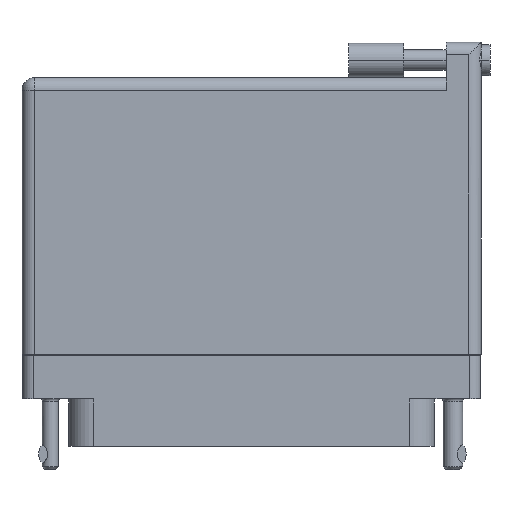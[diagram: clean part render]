
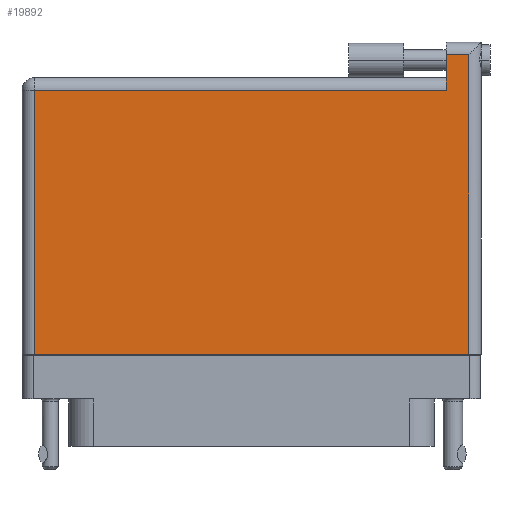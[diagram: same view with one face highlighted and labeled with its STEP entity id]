
A CAD part, front view. The second image highlights one B-rep face of the part: STEP entity #19892.
In plain terms, the highlighted face is planar.
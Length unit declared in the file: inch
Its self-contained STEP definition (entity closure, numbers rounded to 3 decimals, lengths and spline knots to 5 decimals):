
#1408 = CARTESIAN_POINT ( 'NONE',  ( 1.23, 1.666, 0.4495 ) ) ;
#2684 = EDGE_CURVE ( 'NONE', #15771, #12759, #55720, .T. ) ;
#5996 = FACE_OUTER_BOUND ( 'NONE', #47998, .T. ) ;
#6559 = CARTESIAN_POINT ( 'NONE',  ( -1.3, 1.466, 0.4495 ) ) ;
#7021 = EDGE_CURVE ( 'NONE', #54679, #48493, #30972, .T. ) ;
#7186 = VECTOR ( 'NONE', #22180, 39.37008 ) ;
#11133 = VECTOR ( 'NONE', #48648, 39.37008 ) ;
#11405 = CARTESIAN_POINT ( 'NONE',  ( 1.23, 1.596, 0.4495 ) ) ;
#11908 = ORIENTED_EDGE ( 'NONE', *, *, #27529, .T. ) ;
#12759 = VERTEX_POINT ( 'NONE', #29546 ) ;
#13455 = EDGE_CURVE ( 'NONE', #48493, #41974, #55387, .T. ) ;
#15771 = VERTEX_POINT ( 'NONE', #11405 ) ;
#19892 = ADVANCED_FACE ( 'NONE', ( #5996 ), #20481, .F. ) ;
#20481 = PLANE ( 'NONE',  #52859 ) ;
#20877 = ORIENTED_EDGE ( 'NONE', *, *, #7021, .T. ) ;
#22180 = DIRECTION ( 'NONE',  ( -1., 0., 0. ) ) ;
#22475 = ORIENTED_EDGE ( 'NONE', *, *, #58324, .T. ) ;
#27529 = EDGE_CURVE ( 'NONE', #51222, #54679, #41336, .T. ) ;
#28991 = CARTESIAN_POINT ( 'NONE',  ( -1.3, 1.396, 0.4495 ) ) ;
#29499 = CARTESIAN_POINT ( 'NONE',  ( -1.3, -0.1, 0.4495 ) ) ;
#29546 = CARTESIAN_POINT ( 'NONE',  ( 1.103, 1.596, 0.4495 ) ) ;
#29896 = DIRECTION ( 'NONE',  ( 1., 0., 0. ) ) ;
#30972 = LINE ( 'NONE', #33881, #50880 ) ;
#31737 = VECTOR ( 'NONE', #47667, 39.37008 ) ;
#33881 = CARTESIAN_POINT ( 'NONE',  ( -1.23, -0.1, 0.4495 ) ) ;
#38364 = LINE ( 'NONE', #60216, #44228 ) ;
#40346 = CARTESIAN_POINT ( 'NONE',  ( 1.103, 1.396, 0.4495 ) ) ;
#41021 = CARTESIAN_POINT ( 'NONE',  ( -1.23, 1.396, 0.4495 ) ) ;
#41336 = LINE ( 'NONE', #28991, #31737 ) ;
#41974 = VERTEX_POINT ( 'NONE', #44937 ) ;
#42903 = VECTOR ( 'NONE', #29896, 39.37008 ) ;
#43570 = DIRECTION ( 'NONE',  ( 0., -1., 0. ) ) ;
#44228 = VECTOR ( 'NONE', #46209, 39.37008 ) ;
#44307 = ORIENTED_EDGE ( 'NONE', *, *, #13455, .T. ) ;
#44333 = DIRECTION ( 'NONE',  ( -1., 0., 0. ) ) ;
#44937 = CARTESIAN_POINT ( 'NONE',  ( 1.23, -0.1, 0.4495 ) ) ;
#46209 = DIRECTION ( 'NONE',  ( 0., -1., 0. ) ) ;
#47667 = DIRECTION ( 'NONE',  ( -1., 0., 0. ) ) ;
#47998 = EDGE_LOOP ( 'NONE', ( #44307, #58967, #52487, #22475, #11908, #20877 ) ) ;
#48493 = VERTEX_POINT ( 'NONE', #55356 ) ;
#48648 = DIRECTION ( 'NONE',  ( 0., 1., 0. ) ) ;
#50334 = CARTESIAN_POINT ( 'NONE',  ( -1.3, 1.596, 0.4495 ) ) ;
#50776 = LINE ( 'NONE', #1408, #11133 ) ;
#50880 = VECTOR ( 'NONE', #43570, 39.37008 ) ;
#51222 = VERTEX_POINT ( 'NONE', #40346 ) ;
#52487 = ORIENTED_EDGE ( 'NONE', *, *, #2684, .T. ) ;
#52859 = AXIS2_PLACEMENT_3D ( 'NONE', #6559, #58108, #44333 ) ;
#54679 = VERTEX_POINT ( 'NONE', #41021 ) ;
#55356 = CARTESIAN_POINT ( 'NONE',  ( -1.23, -0.1, 0.4495 ) ) ;
#55387 = LINE ( 'NONE', #29499, #42903 ) ;
#55720 = LINE ( 'NONE', #50334, #7186 ) ;
#58108 = DIRECTION ( 'NONE',  ( 0., 0., -1. ) ) ;
#58324 = EDGE_CURVE ( 'NONE', #12759, #51222, #38364, .T. ) ;
#58676 = EDGE_CURVE ( 'NONE', #41974, #15771, #50776, .T. ) ;
#58967 = ORIENTED_EDGE ( 'NONE', *, *, #58676, .T. ) ;
#60216 = CARTESIAN_POINT ( 'NONE',  ( 1.103, 1.666, 0.4495 ) ) ;
